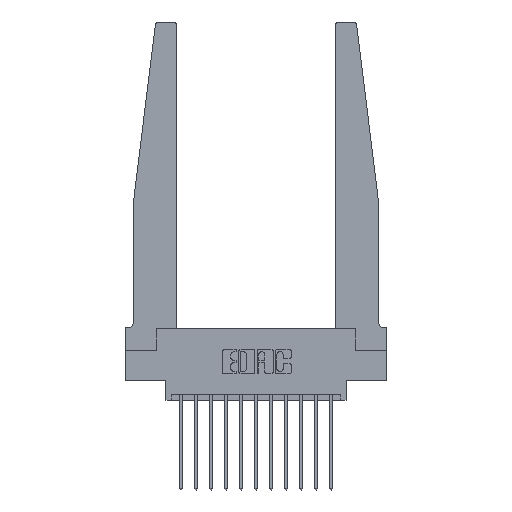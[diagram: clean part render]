
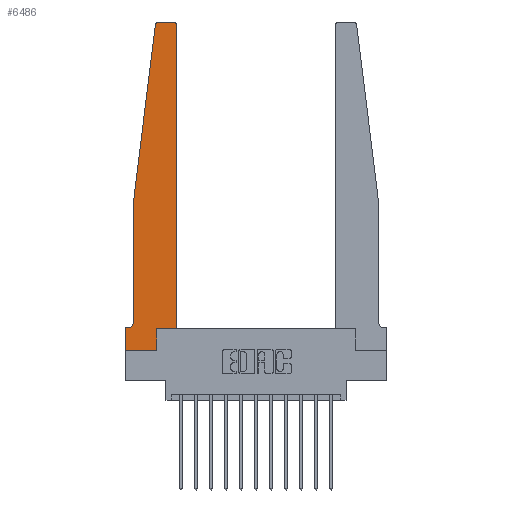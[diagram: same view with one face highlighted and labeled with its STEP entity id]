
A CAD part, top view. The second image highlights one B-rep face of the part: STEP entity #6486.
In plain terms, the highlighted planar face has unit normal (0, 0, 1).
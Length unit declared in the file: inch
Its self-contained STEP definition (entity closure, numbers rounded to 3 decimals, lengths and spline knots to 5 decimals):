
#215 = CARTESIAN_POINT ( 'NONE',  ( 0.2605, 0.18, 0.37 ) ) ;
#509 = PLANE ( 'NONE',  #7949 ) ;
#596 = DIRECTION ( 'NONE',  ( 0., 0., 1. ) ) ;
#642 = LINE ( 'NONE', #8013, #13235 ) ;
#702 = ORIENTED_EDGE ( 'NONE', *, *, #4698, .T. ) ;
#1174 = CARTESIAN_POINT ( 'NONE',  ( 0.395, 2.75, 0.37 ) ) ;
#1499 = LINE ( 'NONE', #215, #4440 ) ;
#1526 = ORIENTED_EDGE ( 'NONE', *, *, #6337, .T. ) ;
#1528 = EDGE_CURVE ( 'NONE', #16090, #10951, #11357, .T. ) ;
#2033 = FACE_OUTER_BOUND ( 'NONE', #9672, .T. ) ;
#2060 = LINE ( 'NONE', #7759, #14630 ) ;
#2123 = ORIENTED_EDGE ( 'NONE', *, *, #10781, .T. ) ;
#2181 = CARTESIAN_POINT ( 'NONE',  ( 0.25, 2.75, 0.37 ) ) ;
#2823 = CARTESIAN_POINT ( 'NONE',  ( 0.2605, 0., 0.37 ) ) ;
#2981 = EDGE_CURVE ( 'NONE', #14205, #16090, #8168, .T. ) ;
#3160 = CARTESIAN_POINT ( 'NONE',  ( 0.27653, 2.75, 0.37 ) ) ;
#3307 = CARTESIAN_POINT ( 'NONE',  ( 0.065, 1.25, 0.37 ) ) ;
#3531 = CARTESIAN_POINT ( 'NONE',  ( 0.425, 0.18, 0.37 ) ) ;
#3763 = LINE ( 'NONE', #8997, #13401 ) ;
#3899 = VECTOR ( 'NONE', #10720, 39.37008 ) ;
#4269 = VERTEX_POINT ( 'NONE', #13344 ) ;
#4358 = CARTESIAN_POINT ( 'NONE',  ( 0.065, 0.1875, 0.37 ) ) ;
#4440 = VECTOR ( 'NONE', #6482, 39.37008 ) ;
#4698 = EDGE_CURVE ( 'NONE', #12687, #7992, #2060, .T. ) ;
#4702 = DIRECTION ( 'NONE',  ( -1., 0., 0. ) ) ;
#4758 = ORIENTED_EDGE ( 'NONE', *, *, #8425, .T. ) ;
#4994 = CARTESIAN_POINT ( 'NONE',  ( 0.24675, 2.72367, 0.37 ) ) ;
#5166 = VERTEX_POINT ( 'NONE', #2823 ) ;
#5352 = DIRECTION ( 'NONE',  ( 0., 0., -1. ) ) ;
#5522 = AXIS2_PLACEMENT_3D ( 'NONE', #12878, #5352, #14142 ) ;
#6337 = EDGE_CURVE ( 'NONE', #10951, #15643, #3763, .T. ) ;
#6482 = DIRECTION ( 'NONE',  ( 0., 1., 0. ) ) ;
#6486 = ADVANCED_FACE ( 'NONE', ( #2033 ), #509, .T. ) ;
#6791 = CARTESIAN_POINT ( 'NONE',  ( 0.27653, 2.72, 0.37 ) ) ;
#6831 = DIRECTION ( 'NONE',  ( 0., 0., 1. ) ) ;
#7174 = ORIENTED_EDGE ( 'NONE', *, *, #9570, .T. ) ;
#7261 = VECTOR ( 'NONE', #13769, 39.37008 ) ;
#7271 = VERTEX_POINT ( 'NONE', #3160 ) ;
#7556 = CARTESIAN_POINT ( 'NONE',  ( 0., 0.1875, 0.37 ) ) ;
#7565 = ORIENTED_EDGE ( 'NONE', *, *, #2981, .T. ) ;
#7759 = CARTESIAN_POINT ( 'NONE',  ( 0.065, 1.25, 0.37 ) ) ;
#7949 = AXIS2_PLACEMENT_3D ( 'NONE', #11840, #6831, #15630 ) ;
#7992 = VERTEX_POINT ( 'NONE', #3307 ) ;
#8013 = CARTESIAN_POINT ( 'NONE',  ( 0., 0., 0.37 ) ) ;
#8036 = DIRECTION ( 'NONE',  ( 1., 0., 0. ) ) ;
#8096 = CARTESIAN_POINT ( 'NONE',  ( 0.395, 2.72, 0.37 ) ) ;
#8168 = CIRCLE ( 'NONE', #5522, 0.05 ) ;
#8224 = CIRCLE ( 'NONE', #12008, 0.03 ) ;
#8235 = EDGE_CURVE ( 'NONE', #4269, #12497, #10594, .T. ) ;
#8425 = EDGE_CURVE ( 'NONE', #7271, #12687, #8224, .T. ) ;
#8535 = DIRECTION ( 'NONE',  ( 1., 0., 0. ) ) ;
#8676 = CARTESIAN_POINT ( 'NONE',  ( 0.425, 0.18, 0.37 ) ) ;
#8978 = ORIENTED_EDGE ( 'NONE', *, *, #8235, .T. ) ;
#8995 = VECTOR ( 'NONE', #4702, 39.37008 ) ;
#8997 = CARTESIAN_POINT ( 'NONE',  ( 0., 0., 0.37 ) ) ;
#9315 = CARTESIAN_POINT ( 'NONE',  ( 0.425, 2.72, 0.37 ) ) ;
#9347 = DIRECTION ( 'NONE',  ( 1., 0., 0. ) ) ;
#9443 = CARTESIAN_POINT ( 'NONE',  ( 0.2605, 0.18, 0.37 ) ) ;
#9549 = ORIENTED_EDGE ( 'NONE', *, *, #11260, .T. ) ;
#9570 = EDGE_CURVE ( 'NONE', #5166, #11829, #1499, .T. ) ;
#9672 = EDGE_LOOP ( 'NONE', ( #12819, #4758, #702, #15631, #7565, #11433, #1526, #13957, #7174, #2123, #8978, #9549 ) ) ;
#10178 = VECTOR ( 'NONE', #15907, 39.37008 ) ;
#10593 = LINE ( 'NONE', #2181, #8995 ) ;
#10594 = LINE ( 'NONE', #8676, #7261 ) ;
#10720 = DIRECTION ( 'NONE',  ( -1., 0., 0. ) ) ;
#10781 = EDGE_CURVE ( 'NONE', #11829, #4269, #15238, .T. ) ;
#10951 = VERTEX_POINT ( 'NONE', #7556 ) ;
#11260 = EDGE_CURVE ( 'NONE', #12497, #16024, #16016, .T. ) ;
#11357 = LINE ( 'NONE', #4358, #3899 ) ;
#11433 = ORIENTED_EDGE ( 'NONE', *, *, #1528, .T. ) ;
#11776 = DIRECTION ( 'NONE',  ( 1., 0., 0. ) ) ;
#11829 = VERTEX_POINT ( 'NONE', #9443 ) ;
#11840 = CARTESIAN_POINT ( 'NONE',  ( 0., 0.1875, 0.37 ) ) ;
#12008 = AXIS2_PLACEMENT_3D ( 'NONE', #6791, #15590, #8036 ) ;
#12292 = VECTOR ( 'NONE', #8535, 39.37008 ) ;
#12423 = EDGE_CURVE ( 'NONE', #15643, #5166, #642, .T. ) ;
#12497 = VERTEX_POINT ( 'NONE', #9315 ) ;
#12687 = VERTEX_POINT ( 'NONE', #4994 ) ;
#12819 = ORIENTED_EDGE ( 'NONE', *, *, #14453, .T. ) ;
#12878 = CARTESIAN_POINT ( 'NONE',  ( 0.015, 0.2375, 0.37 ) ) ;
#13085 = AXIS2_PLACEMENT_3D ( 'NONE', #8096, #596, #9347 ) ;
#13235 = VECTOR ( 'NONE', #11776, 39.37008 ) ;
#13344 = CARTESIAN_POINT ( 'NONE',  ( 0.425, 0.18, 0.37 ) ) ;
#13401 = VECTOR ( 'NONE', #14035, 39.37008 ) ;
#13554 = LINE ( 'NONE', #14641, #10178 ) ;
#13769 = DIRECTION ( 'NONE',  ( 0., 1., 0. ) ) ;
#13803 = CARTESIAN_POINT ( 'NONE',  ( 0.015, 0.1875, 0.37 ) ) ;
#13957 = ORIENTED_EDGE ( 'NONE', *, *, #12423, .T. ) ;
#14035 = DIRECTION ( 'NONE',  ( 0., -1., 0. ) ) ;
#14098 = DIRECTION ( 'NONE',  ( -0.122, -0.992, 0. ) ) ;
#14142 = DIRECTION ( 'NONE',  ( -1., 0., 0. ) ) ;
#14205 = VERTEX_POINT ( 'NONE', #14334 ) ;
#14267 = CARTESIAN_POINT ( 'NONE',  ( 0., 0., 0.37 ) ) ;
#14334 = CARTESIAN_POINT ( 'NONE',  ( 0.065, 0.2375, 0.37 ) ) ;
#14453 = EDGE_CURVE ( 'NONE', #16024, #7271, #10593, .T. ) ;
#14630 = VECTOR ( 'NONE', #14098, 39.37008 ) ;
#14641 = CARTESIAN_POINT ( 'NONE',  ( 0.065, 1.25, 0.37 ) ) ;
#15238 = LINE ( 'NONE', #3531, #12292 ) ;
#15590 = DIRECTION ( 'NONE',  ( 0., 0., 1. ) ) ;
#15630 = DIRECTION ( 'NONE',  ( 1., 0., 0. ) ) ;
#15631 = ORIENTED_EDGE ( 'NONE', *, *, #15846, .T. ) ;
#15643 = VERTEX_POINT ( 'NONE', #14267 ) ;
#15846 = EDGE_CURVE ( 'NONE', #7992, #14205, #13554, .T. ) ;
#15907 = DIRECTION ( 'NONE',  ( 0., -1., 0. ) ) ;
#16016 = CIRCLE ( 'NONE', #13085, 0.03 ) ;
#16024 = VERTEX_POINT ( 'NONE', #1174 ) ;
#16090 = VERTEX_POINT ( 'NONE', #13803 ) ;
